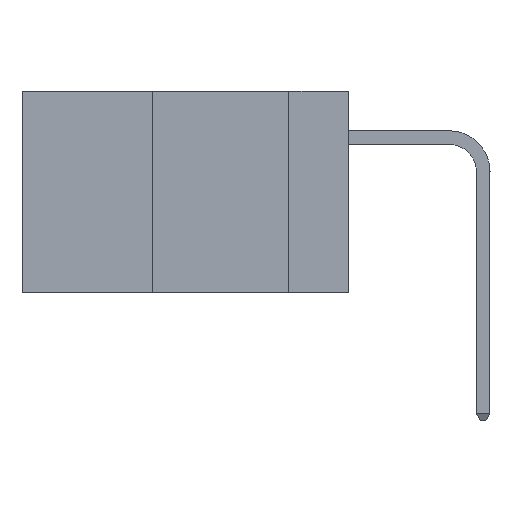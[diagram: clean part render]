
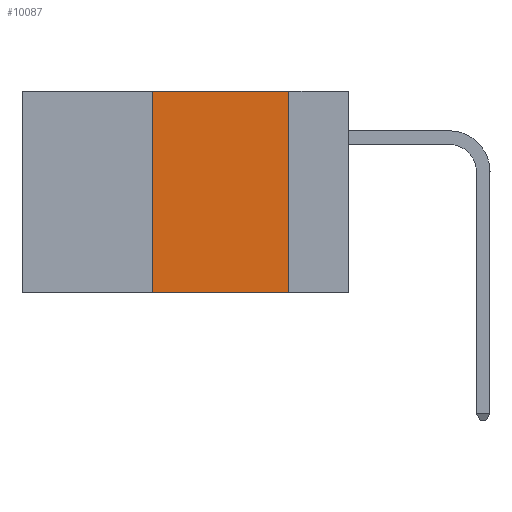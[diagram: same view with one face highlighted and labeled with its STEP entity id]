
A CAD part, left-side view. The second image highlights one B-rep face of the part: STEP entity #10087.
In plain terms, the highlighted planar face has unit normal (-1, 0, 0).
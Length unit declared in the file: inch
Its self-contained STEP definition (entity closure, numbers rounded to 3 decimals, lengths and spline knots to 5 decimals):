
#579 = CARTESIAN_POINT ( 'NONE',  ( 0., 0.6, -0.37 ) ) ;
#1259 = CARTESIAN_POINT ( 'NONE',  ( 0., 0.6, 0. ) ) ;
#3484 = LINE ( 'NONE', #4163, #31419 ) ;
#4096 = DIRECTION ( 'NONE',  ( 0., -1., 0. ) ) ;
#4163 = CARTESIAN_POINT ( 'NONE',  ( 0., 0.36, 0. ) ) ;
#5533 = DIRECTION ( 'NONE',  ( 0., 0., -1. ) ) ;
#6232 = ORIENTED_EDGE ( 'NONE', *, *, #23566, .F. ) ;
#6706 = ORIENTED_EDGE ( 'NONE', *, *, #41470, .F. ) ;
#6926 = VECTOR ( 'NONE', #4096, 39.37008 ) ;
#7072 = VECTOR ( 'NONE', #24687, 39.37008 ) ;
#7817 = AXIS2_PLACEMENT_3D ( 'NONE', #40359, #17896, #30816 ) ;
#10087 = ADVANCED_FACE ( 'NONE', ( #41682 ), #42087, .F. ) ;
#10749 = VERTEX_POINT ( 'NONE', #25387 ) ;
#12100 = VERTEX_POINT ( 'NONE', #26162 ) ;
#17380 = LINE ( 'NONE', #28447, #29771 ) ;
#17896 = DIRECTION ( 'NONE',  ( 1., 0., 0. ) ) ;
#21696 = ORIENTED_EDGE ( 'NONE', *, *, #41974, .T. ) ;
#23315 = EDGE_LOOP ( 'NONE', ( #6706, #6232, #37936, #21696 ) ) ;
#23566 = EDGE_CURVE ( 'NONE', #12100, #10749, #29384, .T. ) ;
#24687 = DIRECTION ( 'NONE',  ( 0., -1., 0. ) ) ;
#25366 = VERTEX_POINT ( 'NONE', #33435 ) ;
#25387 = CARTESIAN_POINT ( 'NONE',  ( 0., 0.11, 0. ) ) ;
#26162 = CARTESIAN_POINT ( 'NONE',  ( 0., 0.36, 0. ) ) ;
#28447 = CARTESIAN_POINT ( 'NONE',  ( 0., 0.11, 0. ) ) ;
#29384 = LINE ( 'NONE', #1259, #7072 ) ;
#29438 = VERTEX_POINT ( 'NONE', #37971 ) ;
#29771 = VECTOR ( 'NONE', #5533, 39.37008 ) ;
#30816 = DIRECTION ( 'NONE',  ( 0., 0., -1. ) ) ;
#31419 = VECTOR ( 'NONE', #33838, 39.37008 ) ;
#33435 = CARTESIAN_POINT ( 'NONE',  ( 0., 0.11, -0.37 ) ) ;
#33838 = DIRECTION ( 'NONE',  ( 0., 0., 1. ) ) ;
#37936 = ORIENTED_EDGE ( 'NONE', *, *, #40144, .F. ) ;
#37971 = CARTESIAN_POINT ( 'NONE',  ( 0., 0.36, -0.37 ) ) ;
#40107 = LINE ( 'NONE', #579, #6926 ) ;
#40144 = EDGE_CURVE ( 'NONE', #29438, #12100, #3484, .T. ) ;
#40359 = CARTESIAN_POINT ( 'NONE',  ( 0., 0.6, 0. ) ) ;
#41470 = EDGE_CURVE ( 'NONE', #10749, #25366, #17380, .T. ) ;
#41682 = FACE_OUTER_BOUND ( 'NONE', #23315, .T. ) ;
#41974 = EDGE_CURVE ( 'NONE', #29438, #25366, #40107, .T. ) ;
#42087 = PLANE ( 'NONE',  #7817 ) ;
